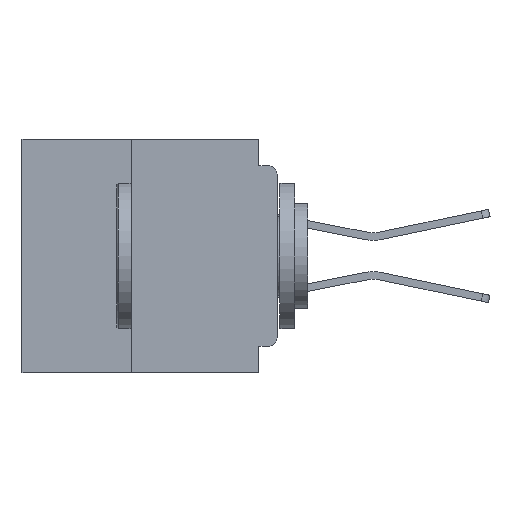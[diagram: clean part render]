
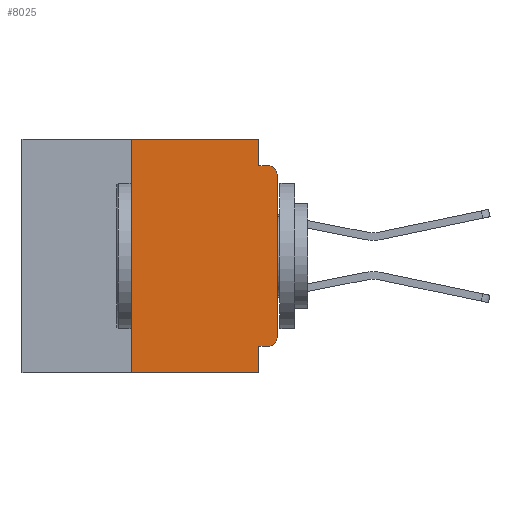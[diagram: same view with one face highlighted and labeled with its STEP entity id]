
A CAD part, left-side view. The second image highlights one B-rep face of the part: STEP entity #8025.
In plain terms, the highlighted planar face has unit normal (-1, 0, 0).
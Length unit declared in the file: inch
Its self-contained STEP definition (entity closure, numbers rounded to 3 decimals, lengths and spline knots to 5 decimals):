
#1481 = DIRECTION ( 'NONE',  ( 0., 0., 1. ) ) ;
#1595 = EDGE_CURVE ( 'NONE', #11669, #4816, #19228, .T. ) ;
#1869 = VERTEX_POINT ( 'NONE', #28713 ) ;
#2038 = DIRECTION ( 'NONE',  ( 1., 0., 0. ) ) ;
#2661 = VECTOR ( 'NONE', #6537, 39.37008 ) ;
#3082 = ORIENTED_EDGE ( 'NONE', *, *, #8282, .F. ) ;
#4816 = VERTEX_POINT ( 'NONE', #34003 ) ;
#4862 = AXIS2_PLACEMENT_3D ( 'NONE', #18066, #39026, #21111 ) ;
#5486 = LINE ( 'NONE', #12473, #29479 ) ;
#5561 = CARTESIAN_POINT ( 'NONE',  ( 0., 0.031, -0.045 ) ) ;
#6311 = CARTESIAN_POINT ( 'NONE',  ( 0., 0., -0.045 ) ) ;
#6537 = DIRECTION ( 'NONE',  ( 0., 0., 1. ) ) ;
#6713 = CARTESIAN_POINT ( 'NONE',  ( 0., 0., -0.06 ) ) ;
#6986 = FACE_OUTER_BOUND ( 'NONE', #36780, .T. ) ;
#7577 = CARTESIAN_POINT ( 'NONE',  ( 0., 0.031, -0.4 ) ) ;
#7640 = LINE ( 'NONE', #19015, #31558 ) ;
#7708 = VERTEX_POINT ( 'NONE', #6713 ) ;
#7758 = VECTOR ( 'NONE', #18303, 39.37008 ) ;
#7770 = CARTESIAN_POINT ( 'NONE',  ( 0., 0.437, 0. ) ) ;
#7930 = VERTEX_POINT ( 'NONE', #34721 ) ;
#8025 = ADVANCED_FACE ( 'NONE', ( #6986 ), #14189, .F. ) ;
#8198 = CARTESIAN_POINT ( 'NONE',  ( 0., 0.437, 0. ) ) ;
#8282 = EDGE_CURVE ( 'NONE', #26819, #38220, #5486, .T. ) ;
#9269 = VERTEX_POINT ( 'NONE', #32790 ) ;
#9721 = LINE ( 'NONE', #19597, #31752 ) ;
#10106 = ORIENTED_EDGE ( 'NONE', *, *, #17282, .F. ) ;
#10319 = VECTOR ( 'NONE', #1481, 39.37008 ) ;
#10421 = CARTESIAN_POINT ( 'NONE',  ( 0., 0.031, -0.355 ) ) ;
#10816 = DIRECTION ( 'NONE',  ( 0., -1., 0. ) ) ;
#11669 = VERTEX_POINT ( 'NONE', #25209 ) ;
#12473 = CARTESIAN_POINT ( 'NONE',  ( 0., 0.031, 0. ) ) ;
#13780 = ORIENTED_EDGE ( 'NONE', *, *, #32924, .T. ) ;
#14189 = PLANE ( 'NONE',  #16482 ) ;
#14421 = CARTESIAN_POINT ( 'NONE',  ( 0., 0.015, -0.06 ) ) ;
#15882 = LINE ( 'NONE', #7577, #38852 ) ;
#16049 = ORIENTED_EDGE ( 'NONE', *, *, #24569, .F. ) ;
#16482 = AXIS2_PLACEMENT_3D ( 'NONE', #8198, #2038, #23234 ) ;
#17282 = EDGE_CURVE ( 'NONE', #7930, #21323, #9721, .T. ) ;
#17427 = DIRECTION ( 'NONE',  ( 0., 0., -1. ) ) ;
#18066 = CARTESIAN_POINT ( 'NONE',  ( 0., 0.015, -0.34 ) ) ;
#18303 = DIRECTION ( 'NONE',  ( 0., -1., 0. ) ) ;
#18513 = VERTEX_POINT ( 'NONE', #33567 ) ;
#19015 = CARTESIAN_POINT ( 'NONE',  ( 0., 0.437, -0.4 ) ) ;
#19228 = LINE ( 'NONE', #31631, #10319 ) ;
#19597 = CARTESIAN_POINT ( 'NONE',  ( 0., 0., -0.355 ) ) ;
#21111 = DIRECTION ( 'NONE',  ( 0., 0., -1. ) ) ;
#21323 = VERTEX_POINT ( 'NONE', #10421 ) ;
#21400 = DIRECTION ( 'NONE',  ( 0., 0., -1. ) ) ;
#21432 = ORIENTED_EDGE ( 'NONE', *, *, #1595, .F. ) ;
#23234 = DIRECTION ( 'NONE',  ( 0., 0., -1. ) ) ;
#23300 = ORIENTED_EDGE ( 'NONE', *, *, #38157, .T. ) ;
#23612 = LINE ( 'NONE', #7770, #38620 ) ;
#24526 = CARTESIAN_POINT ( 'NONE',  ( 0., 0., 0. ) ) ;
#24569 = EDGE_CURVE ( 'NONE', #38220, #1869, #31682, .T. ) ;
#24614 = CIRCLE ( 'NONE', #4862, 0.015 ) ;
#24860 = ORIENTED_EDGE ( 'NONE', *, *, #36836, .F. ) ;
#25209 = CARTESIAN_POINT ( 'NONE',  ( 0., 0.25, -0.4 ) ) ;
#26819 = VERTEX_POINT ( 'NONE', #32493 ) ;
#27981 = ORIENTED_EDGE ( 'NONE', *, *, #35938, .T. ) ;
#28713 = CARTESIAN_POINT ( 'NONE',  ( 0., 0.015, -0.045 ) ) ;
#29479 = VECTOR ( 'NONE', #21400, 39.37008 ) ;
#29721 = ORIENTED_EDGE ( 'NONE', *, *, #38501, .T. ) ;
#30924 = DIRECTION ( 'NONE',  ( 0., -1., 0. ) ) ;
#31558 = VECTOR ( 'NONE', #30924, 39.37008 ) ;
#31566 = DIRECTION ( 'NONE',  ( 0., 0., -1. ) ) ;
#31631 = CARTESIAN_POINT ( 'NONE',  ( 0., 0.25, -0.4 ) ) ;
#31682 = LINE ( 'NONE', #6311, #7758 ) ;
#31752 = VECTOR ( 'NONE', #37545, 39.37008 ) ;
#32141 = ORIENTED_EDGE ( 'NONE', *, *, #38041, .F. ) ;
#32493 = CARTESIAN_POINT ( 'NONE',  ( 0., 0.031, 0. ) ) ;
#32790 = CARTESIAN_POINT ( 'NONE',  ( 0., 0.031, -0.4 ) ) ;
#32924 = EDGE_CURVE ( 'NONE', #7930, #18513, #24614, .T. ) ;
#33567 = CARTESIAN_POINT ( 'NONE',  ( 0., 0., -0.34 ) ) ;
#33967 = CIRCLE ( 'NONE', #36540, 0.015 ) ;
#34003 = CARTESIAN_POINT ( 'NONE',  ( 0., 0.25, 0. ) ) ;
#34721 = CARTESIAN_POINT ( 'NONE',  ( 0., 0.015, -0.355 ) ) ;
#34839 = LINE ( 'NONE', #24526, #2661 ) ;
#35460 = DIRECTION ( 'NONE',  ( -1., 0., 0. ) ) ;
#35938 = EDGE_CURVE ( 'NONE', #18513, #7708, #34839, .T. ) ;
#36540 = AXIS2_PLACEMENT_3D ( 'NONE', #14421, #35460, #17427 ) ;
#36780 = EDGE_LOOP ( 'NONE', ( #27981, #23300, #16049, #3082, #32141, #21432, #29721, #24860, #10106, #13780 ) ) ;
#36836 = EDGE_CURVE ( 'NONE', #21323, #9269, #15882, .T. ) ;
#37545 = DIRECTION ( 'NONE',  ( 0., 1., 0. ) ) ;
#38041 = EDGE_CURVE ( 'NONE', #4816, #26819, #23612, .T. ) ;
#38157 = EDGE_CURVE ( 'NONE', #7708, #1869, #33967, .T. ) ;
#38220 = VERTEX_POINT ( 'NONE', #5561 ) ;
#38501 = EDGE_CURVE ( 'NONE', #11669, #9269, #7640, .T. ) ;
#38620 = VECTOR ( 'NONE', #10816, 39.37008 ) ;
#38852 = VECTOR ( 'NONE', #31566, 39.37008 ) ;
#39026 = DIRECTION ( 'NONE',  ( -1., 0., 0. ) ) ;
